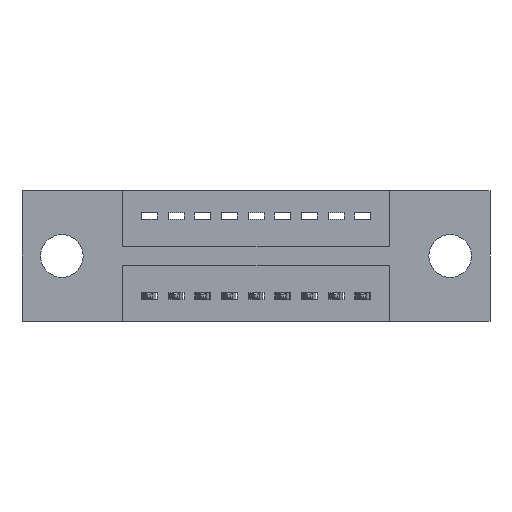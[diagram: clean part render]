
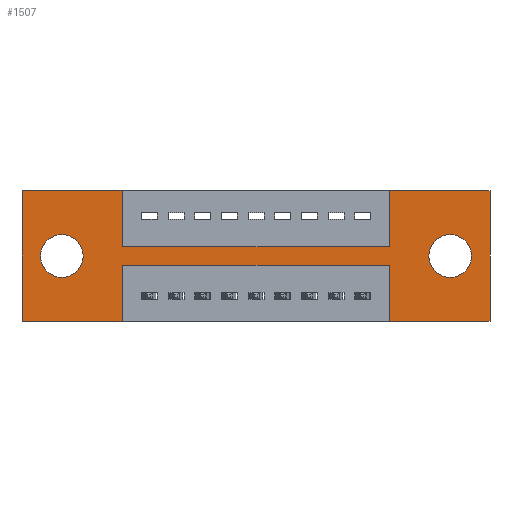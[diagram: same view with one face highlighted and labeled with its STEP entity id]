
A CAD part, front view. The second image highlights one B-rep face of the part: STEP entity #1507.
In plain terms, the highlighted planar face has unit normal (0, -1, 0).
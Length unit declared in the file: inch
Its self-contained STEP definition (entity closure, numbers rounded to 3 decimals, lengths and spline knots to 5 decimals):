
#138 = DIRECTION ( 'NONE',  ( 1., 0., 0. ) ) ;
#336 = CARTESIAN_POINT ( 'NONE',  ( 0.3775, 0., -0.49 ) ) ;
#481 = CARTESIAN_POINT ( 'NONE',  ( 1.6055, 0., -0.245 ) ) ;
#500 = VERTEX_POINT ( 'NONE', #9368 ) ;
#551 = VERTEX_POINT ( 'NONE', #9278 ) ;
#557 = EDGE_CURVE ( 'NONE', #551, #8829, #987, .T. ) ;
#625 = FACE_BOUND ( 'NONE', #1404, .T. ) ;
#650 = ORIENTED_EDGE ( 'NONE', *, *, #3277, .T. ) ;
#670 = CARTESIAN_POINT ( 'NONE',  ( 0., 0., -0.49 ) ) ;
#678 = EDGE_CURVE ( 'NONE', #1936, #3964, #8015, .T. ) ;
#781 = ORIENTED_EDGE ( 'NONE', *, *, #6232, .F. ) ;
#819 = ORIENTED_EDGE ( 'NONE', *, *, #678, .F. ) ;
#905 = ORIENTED_EDGE ( 'NONE', *, *, #9582, .T. ) ;
#987 = LINE ( 'NONE', #7048, #2176 ) ;
#999 = CARTESIAN_POINT ( 'NONE',  ( 0., 0., 0. ) ) ;
#1071 = VERTEX_POINT ( 'NONE', #2089 ) ;
#1075 = CARTESIAN_POINT ( 'NONE',  ( 0., 0., 0. ) ) ;
#1091 = FACE_BOUND ( 'NONE', #3006, .T. ) ;
#1124 = CARTESIAN_POINT ( 'NONE',  ( 0., 0., -0.49 ) ) ;
#1217 = CIRCLE ( 'NONE', #5800, 0.08 ) ;
#1404 = EDGE_LOOP ( 'NONE', ( #5078, #9369 ) ) ;
#1440 = VECTOR ( 'NONE', #9559, 39.37008 ) ;
#1482 = VERTEX_POINT ( 'NONE', #3357 ) ;
#1507 = ADVANCED_FACE ( 'NONE', ( #1091, #625, #6531 ), #4855, .T. ) ;
#1576 = DIRECTION ( 'NONE',  ( 0., 0., 1. ) ) ;
#1608 = VERTEX_POINT ( 'NONE', #3317 ) ;
#1679 = LINE ( 'NONE', #4986, #7999 ) ;
#1779 = EDGE_CURVE ( 'NONE', #3181, #2291, #9123, .T. ) ;
#1810 = CARTESIAN_POINT ( 'NONE',  ( 1.6055, 0., -0.245 ) ) ;
#1811 = DIRECTION ( 'NONE',  ( 1., 0., 0. ) ) ;
#1886 = CARTESIAN_POINT ( 'NONE',  ( 0.3775, 0., -0.28 ) ) ;
#1936 = VERTEX_POINT ( 'NONE', #8241 ) ;
#1943 = DIRECTION ( 'NONE',  ( 0., 1., 0. ) ) ;
#2002 = LINE ( 'NONE', #3316, #3075 ) ;
#2089 = CARTESIAN_POINT ( 'NONE',  ( 1.3775, 0., -0.28 ) ) ;
#2117 = EDGE_CURVE ( 'NONE', #1071, #1936, #3460, .T. ) ;
#2176 = VECTOR ( 'NONE', #1811, 39.37008 ) ;
#2291 = VERTEX_POINT ( 'NONE', #5908 ) ;
#2375 = EDGE_CURVE ( 'NONE', #500, #1071, #5463, .T. ) ;
#2508 = EDGE_LOOP ( 'NONE', ( #6097, #3368, #5213, #8708, #9205, #9274, #819, #3240, #2892, #781, #5507, #9521 ) ) ;
#2574 = CARTESIAN_POINT ( 'NONE',  ( 0., 0., -0.49 ) ) ;
#2745 = VECTOR ( 'NONE', #6410, 39.37008 ) ;
#2892 = ORIENTED_EDGE ( 'NONE', *, *, #2375, .F. ) ;
#2946 = CARTESIAN_POINT ( 'NONE',  ( 1.6055, 0., -0.165 ) ) ;
#2962 = VERTEX_POINT ( 'NONE', #670 ) ;
#3006 = EDGE_LOOP ( 'NONE', ( #650, #905 ) ) ;
#3057 = CARTESIAN_POINT ( 'NONE',  ( 0., 0., 0. ) ) ;
#3075 = VECTOR ( 'NONE', #5804, 39.37008 ) ;
#3181 = VERTEX_POINT ( 'NONE', #9204 ) ;
#3240 = ORIENTED_EDGE ( 'NONE', *, *, #2117, .F. ) ;
#3277 = EDGE_CURVE ( 'NONE', #8340, #1482, #8660, .T. ) ;
#3316 = CARTESIAN_POINT ( 'NONE',  ( 1.3775, 0., -0.21 ) ) ;
#3317 = CARTESIAN_POINT ( 'NONE',  ( 1.755, 0., -0.49 ) ) ;
#3357 = CARTESIAN_POINT ( 'NONE',  ( 1.6055, 0., -0.325 ) ) ;
#3368 = ORIENTED_EDGE ( 'NONE', *, *, #557, .F. ) ;
#3444 = VECTOR ( 'NONE', #138, 39.37008 ) ;
#3451 = DIRECTION ( 'NONE',  ( 0., 0., -1. ) ) ;
#3460 = LINE ( 'NONE', #6369, #1440 ) ;
#3492 = AXIS2_PLACEMENT_3D ( 'NONE', #2574, #4119, #4891 ) ;
#3660 = CARTESIAN_POINT ( 'NONE',  ( 1.3775, 0., -0.28 ) ) ;
#3964 = VERTEX_POINT ( 'NONE', #336 ) ;
#3970 = VECTOR ( 'NONE', #3451, 39.37008 ) ;
#4103 = LINE ( 'NONE', #1124, #7052 ) ;
#4119 = DIRECTION ( 'NONE',  ( 0., -1., 0. ) ) ;
#4424 = VERTEX_POINT ( 'NONE', #5447 ) ;
#4441 = VERTEX_POINT ( 'NONE', #8537 ) ;
#4492 = EDGE_CURVE ( 'NONE', #4441, #9705, #5117, .T. ) ;
#4575 = DIRECTION ( 'NONE',  ( 1., 0., 0. ) ) ;
#4640 = EDGE_CURVE ( 'NONE', #8829, #4441, #2002, .T. ) ;
#4770 = CARTESIAN_POINT ( 'NONE',  ( 0.1495, 0., -0.245 ) ) ;
#4855 = PLANE ( 'NONE',  #3492 ) ;
#4870 = DIRECTION ( 'NONE',  ( -1., 0., 0. ) ) ;
#4891 = DIRECTION ( 'NONE',  ( 0., 0., -1. ) ) ;
#4986 = CARTESIAN_POINT ( 'NONE',  ( 0., 0., -0.49 ) ) ;
#5078 = ORIENTED_EDGE ( 'NONE', *, *, #9543, .T. ) ;
#5098 = VECTOR ( 'NONE', #9558, 39.37008 ) ;
#5117 = LINE ( 'NONE', #999, #3444 ) ;
#5190 = EDGE_CURVE ( 'NONE', #2291, #551, #6254, .T. ) ;
#5213 = ORIENTED_EDGE ( 'NONE', *, *, #5190, .F. ) ;
#5416 = LINE ( 'NONE', #1075, #7309 ) ;
#5447 = CARTESIAN_POINT ( 'NONE',  ( 0.1495, 0., -0.325 ) ) ;
#5463 = LINE ( 'NONE', #3660, #9221 ) ;
#5507 = ORIENTED_EDGE ( 'NONE', *, *, #7899, .F. ) ;
#5737 = DIRECTION ( 'NONE',  ( -1., 0., 0. ) ) ;
#5800 = AXIS2_PLACEMENT_3D ( 'NONE', #6442, #7248, #9509 ) ;
#5804 = DIRECTION ( 'NONE',  ( 0., 0., 1. ) ) ;
#5908 = CARTESIAN_POINT ( 'NONE',  ( 0.3775, 0., 0. ) ) ;
#6097 = ORIENTED_EDGE ( 'NONE', *, *, #4640, .F. ) ;
#6232 = EDGE_CURVE ( 'NONE', #1608, #500, #4103, .T. ) ;
#6254 = LINE ( 'NONE', #9426, #5098 ) ;
#6369 = CARTESIAN_POINT ( 'NONE',  ( 0.3775, 0., -0.28 ) ) ;
#6410 = DIRECTION ( 'NONE',  ( 0., 0., -1. ) ) ;
#6442 = CARTESIAN_POINT ( 'NONE',  ( 0.1495, 0., -0.245 ) ) ;
#6531 = FACE_OUTER_BOUND ( 'NONE', #2508, .T. ) ;
#6810 = AXIS2_PLACEMENT_3D ( 'NONE', #481, #1943, #8781 ) ;
#7048 = CARTESIAN_POINT ( 'NONE',  ( 0.3775, 0., -0.21 ) ) ;
#7052 = VECTOR ( 'NONE', #4870, 39.37008 ) ;
#7144 = DIRECTION ( 'NONE',  ( 0., 0., -1. ) ) ;
#7248 = DIRECTION ( 'NONE',  ( 0., 1., 0. ) ) ;
#7309 = VECTOR ( 'NONE', #7809, 39.37008 ) ;
#7621 = CARTESIAN_POINT ( 'NONE',  ( 1.3775, 0., -0.21 ) ) ;
#7627 = CIRCLE ( 'NONE', #6810, 0.08 ) ;
#7809 = DIRECTION ( 'NONE',  ( 0., 0., 1. ) ) ;
#7810 = DIRECTION ( 'NONE',  ( 0., 1., 0. ) ) ;
#7899 = EDGE_CURVE ( 'NONE', #9705, #1608, #8791, .T. ) ;
#7969 = EDGE_CURVE ( 'NONE', #3964, #2962, #1679, .T. ) ;
#7978 = CARTESIAN_POINT ( 'NONE',  ( 0.1495, 0., -0.165 ) ) ;
#7999 = VECTOR ( 'NONE', #5737, 39.37008 ) ;
#8015 = LINE ( 'NONE', #1886, #3970 ) ;
#8194 = AXIS2_PLACEMENT_3D ( 'NONE', #1810, #7810, #7144 ) ;
#8241 = CARTESIAN_POINT ( 'NONE',  ( 0.3775, 0., -0.28 ) ) ;
#8340 = VERTEX_POINT ( 'NONE', #2946 ) ;
#8537 = CARTESIAN_POINT ( 'NONE',  ( 1.3775, 0., 0. ) ) ;
#8601 = EDGE_CURVE ( 'NONE', #2962, #3181, #5416, .T. ) ;
#8660 = CIRCLE ( 'NONE', #8194, 0.08 ) ;
#8708 = ORIENTED_EDGE ( 'NONE', *, *, #1779, .F. ) ;
#8781 = DIRECTION ( 'NONE',  ( 0., 0., -1. ) ) ;
#8791 = LINE ( 'NONE', #9526, #2745 ) ;
#8829 = VERTEX_POINT ( 'NONE', #7621 ) ;
#8883 = VECTOR ( 'NONE', #4575, 39.37008 ) ;
#8905 = CARTESIAN_POINT ( 'NONE',  ( 1.755, 0., 0. ) ) ;
#8962 = DIRECTION ( 'NONE',  ( 0., 0., 1. ) ) ;
#9123 = LINE ( 'NONE', #3057, #8883 ) ;
#9194 = VERTEX_POINT ( 'NONE', #7978 ) ;
#9204 = CARTESIAN_POINT ( 'NONE',  ( 0., 0., 0. ) ) ;
#9205 = ORIENTED_EDGE ( 'NONE', *, *, #8601, .F. ) ;
#9221 = VECTOR ( 'NONE', #8962, 39.37008 ) ;
#9274 = ORIENTED_EDGE ( 'NONE', *, *, #7969, .F. ) ;
#9278 = CARTESIAN_POINT ( 'NONE',  ( 0.3775, 0., -0.21 ) ) ;
#9362 = DIRECTION ( 'NONE',  ( 0., 1., 0. ) ) ;
#9368 = CARTESIAN_POINT ( 'NONE',  ( 1.3775, 0., -0.49 ) ) ;
#9369 = ORIENTED_EDGE ( 'NONE', *, *, #9530, .T. ) ;
#9426 = CARTESIAN_POINT ( 'NONE',  ( 0.3775, 0., -0.21 ) ) ;
#9509 = DIRECTION ( 'NONE',  ( 0., 0., 1. ) ) ;
#9521 = ORIENTED_EDGE ( 'NONE', *, *, #4492, .F. ) ;
#9526 = CARTESIAN_POINT ( 'NONE',  ( 1.755, 0., 0. ) ) ;
#9530 = EDGE_CURVE ( 'NONE', #4424, #9194, #9602, .T. ) ;
#9543 = EDGE_CURVE ( 'NONE', #9194, #4424, #1217, .T. ) ;
#9558 = DIRECTION ( 'NONE',  ( 0., 0., -1. ) ) ;
#9559 = DIRECTION ( 'NONE',  ( -1., 0., 0. ) ) ;
#9582 = EDGE_CURVE ( 'NONE', #1482, #8340, #7627, .T. ) ;
#9602 = CIRCLE ( 'NONE', #9658, 0.08 ) ;
#9658 = AXIS2_PLACEMENT_3D ( 'NONE', #4770, #9362, #1576 ) ;
#9705 = VERTEX_POINT ( 'NONE', #8905 ) ;
